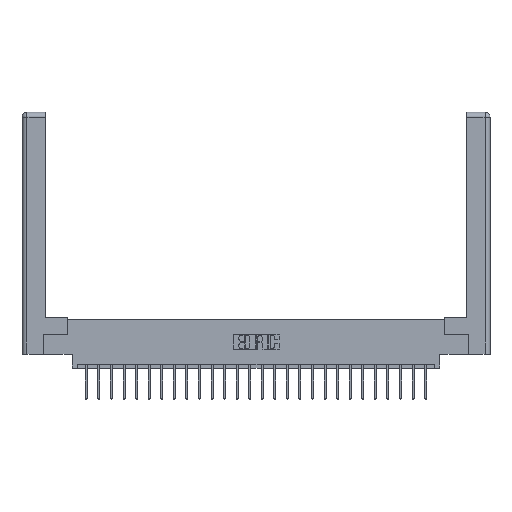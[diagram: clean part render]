
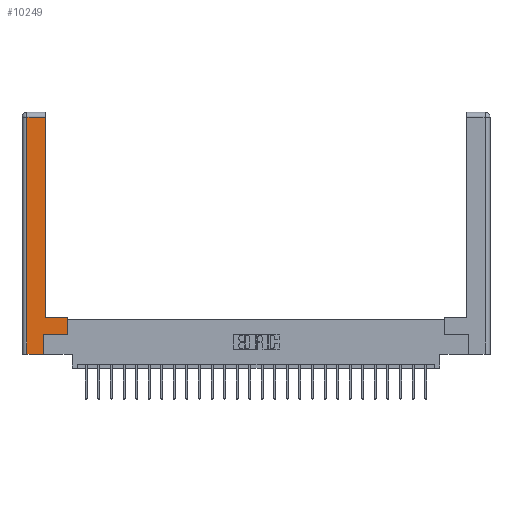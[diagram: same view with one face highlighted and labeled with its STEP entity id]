
A CAD part, top view. The second image highlights one B-rep face of the part: STEP entity #10249.
In plain terms, the highlighted planar face has unit normal (0, 0, 1).
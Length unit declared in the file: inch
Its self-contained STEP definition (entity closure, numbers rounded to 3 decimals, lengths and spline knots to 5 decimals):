
#1678 = ORIENTED_EDGE ( 'NONE', *, *, #23086, .T. ) ;
#1937 = ORIENTED_EDGE ( 'NONE', *, *, #16808, .T. ) ;
#2066 = DIRECTION ( 'NONE',  ( 0., 1., 0. ) ) ;
#3022 = FACE_OUTER_BOUND ( 'NONE', #7716, .T. ) ;
#3368 = CARTESIAN_POINT ( 'NONE',  ( 0.565, 0.245, 0. ) ) ;
#4451 = VECTOR ( 'NONE', #2066, 39.37008 ) ;
#4930 = ORIENTED_EDGE ( 'NONE', *, *, #9945, .T. ) ;
#5952 = DIRECTION ( 'NONE',  ( 0., 1., 0. ) ) ;
#6153 = CARTESIAN_POINT ( 'NONE',  ( 0.265, 0.245, 0. ) ) ;
#6264 = VECTOR ( 'NONE', #7832, 39.37008 ) ;
#6566 = PLANE ( 'NONE',  #8169 ) ;
#6657 = VECTOR ( 'NONE', #12230, 39.37008 ) ;
#7254 = VERTEX_POINT ( 'NONE', #7824 ) ;
#7716 = EDGE_LOOP ( 'NONE', ( #9444, #12898, #1678, #15384, #21171, #1937, #11843, #4930 ) ) ;
#7824 = CARTESIAN_POINT ( 'NONE',  ( 0.565, 0.245, 0. ) ) ;
#7832 = DIRECTION ( 'NONE',  ( -1., 0., 0. ) ) ;
#7992 = CARTESIAN_POINT ( 'NONE',  ( 0.565, 0.45, 0. ) ) ;
#8169 = AXIS2_PLACEMENT_3D ( 'NONE', #21007, #8681, #22882 ) ;
#8520 = EDGE_CURVE ( 'NONE', #11245, #18897, #17069, .T. ) ;
#8652 = CARTESIAN_POINT ( 'NONE',  ( 0.295, 0.45, 0. ) ) ;
#8681 = DIRECTION ( 'NONE',  ( 0., 0., -1. ) ) ;
#9444 = ORIENTED_EDGE ( 'NONE', *, *, #17581, .T. ) ;
#9531 = VERTEX_POINT ( 'NONE', #21088 ) ;
#9945 = EDGE_CURVE ( 'NONE', #21499, #18402, #14514, .T. ) ;
#9967 = CARTESIAN_POINT ( 'NONE',  ( 0.0615, 2.94, 0. ) ) ;
#10065 = VECTOR ( 'NONE', #25262, 39.37008 ) ;
#10249 = ADVANCED_FACE ( 'NONE', ( #3022 ), #6566, .F. ) ;
#10343 = VECTOR ( 'NONE', #13270, 39.37008 ) ;
#10529 = LINE ( 'NONE', #24144, #4451 ) ;
#11245 = VERTEX_POINT ( 'NONE', #16863 ) ;
#11622 = LINE ( 'NONE', #19265, #10343 ) ;
#11843 = ORIENTED_EDGE ( 'NONE', *, *, #13192, .T. ) ;
#12058 = EDGE_CURVE ( 'NONE', #20505, #20466, #10529, .T. ) ;
#12230 = DIRECTION ( 'NONE',  ( 0., -1., 0. ) ) ;
#12406 = CARTESIAN_POINT ( 'NONE',  ( 0.265, 0., 0. ) ) ;
#12898 = ORIENTED_EDGE ( 'NONE', *, *, #8520, .T. ) ;
#13192 = EDGE_CURVE ( 'NONE', #7254, #21499, #21886, .T. ) ;
#13270 = DIRECTION ( 'NONE',  ( 1., 0., 0. ) ) ;
#13786 = LINE ( 'NONE', #3368, #20776 ) ;
#14425 = CARTESIAN_POINT ( 'NONE',  ( 0.0615, 0., 0. ) ) ;
#14514 = LINE ( 'NONE', #8652, #10065 ) ;
#15312 = VECTOR ( 'NONE', #17175, 39.37008 ) ;
#15384 = ORIENTED_EDGE ( 'NONE', *, *, #19741, .T. ) ;
#15955 = LINE ( 'NONE', #21042, #15312 ) ;
#16808 = EDGE_CURVE ( 'NONE', #20466, #7254, #13786, .T. ) ;
#16863 = CARTESIAN_POINT ( 'NONE',  ( 0.295, 2.94, 0. ) ) ;
#17069 = LINE ( 'NONE', #9967, #6264 ) ;
#17175 = DIRECTION ( 'NONE',  ( 0., 1., 0. ) ) ;
#17581 = EDGE_CURVE ( 'NONE', #18402, #11245, #15955, .T. ) ;
#18402 = VERTEX_POINT ( 'NONE', #19872 ) ;
#18897 = VERTEX_POINT ( 'NONE', #25442 ) ;
#19265 = CARTESIAN_POINT ( 'NONE',  ( 0.265, 0., 0. ) ) ;
#19741 = EDGE_CURVE ( 'NONE', #9531, #20505, #11622, .T. ) ;
#19872 = CARTESIAN_POINT ( 'NONE',  ( 0.295, 0.45, 0. ) ) ;
#20466 = VERTEX_POINT ( 'NONE', #6153 ) ;
#20505 = VERTEX_POINT ( 'NONE', #12406 ) ;
#20776 = VECTOR ( 'NONE', #21716, 39.37008 ) ;
#21007 = CARTESIAN_POINT ( 'NONE',  ( 0., 0., 0. ) ) ;
#21042 = CARTESIAN_POINT ( 'NONE',  ( 0.295, 3., 0. ) ) ;
#21088 = CARTESIAN_POINT ( 'NONE',  ( 0.0615, 0., 0. ) ) ;
#21171 = ORIENTED_EDGE ( 'NONE', *, *, #12058, .T. ) ;
#21499 = VERTEX_POINT ( 'NONE', #7992 ) ;
#21716 = DIRECTION ( 'NONE',  ( 1., 0., 0. ) ) ;
#21886 = LINE ( 'NONE', #26093, #24132 ) ;
#22882 = DIRECTION ( 'NONE',  ( -1., 0., 0. ) ) ;
#23086 = EDGE_CURVE ( 'NONE', #18897, #9531, #23862, .T. ) ;
#23862 = LINE ( 'NONE', #14425, #6657 ) ;
#24132 = VECTOR ( 'NONE', #5952, 39.37008 ) ;
#24144 = CARTESIAN_POINT ( 'NONE',  ( 0.265, 0.245, 0. ) ) ;
#25262 = DIRECTION ( 'NONE',  ( -1., 0., 0. ) ) ;
#25442 = CARTESIAN_POINT ( 'NONE',  ( 0.0615, 2.94, 0. ) ) ;
#26093 = CARTESIAN_POINT ( 'NONE',  ( 0.565, 0.45, 0. ) ) ;
